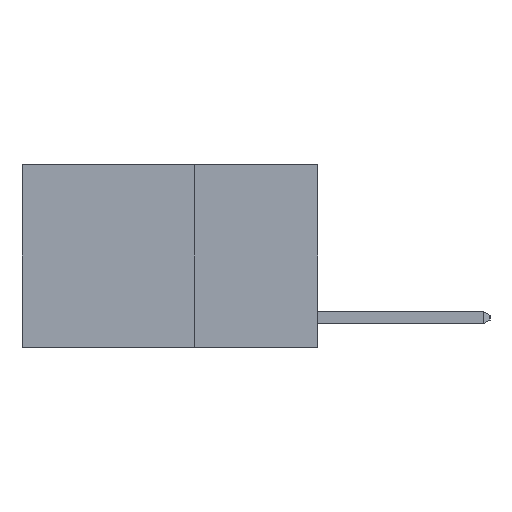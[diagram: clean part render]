
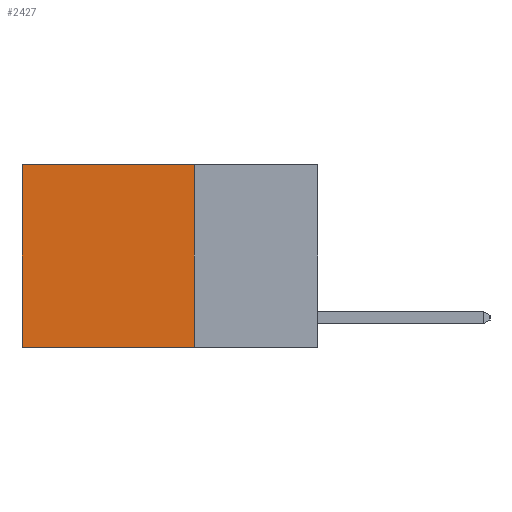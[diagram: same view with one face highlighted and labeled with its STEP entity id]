
A CAD part, left-side view. The second image highlights one B-rep face of the part: STEP entity #2427.
In plain terms, the highlighted planar face has unit normal (-1, 0, 0).
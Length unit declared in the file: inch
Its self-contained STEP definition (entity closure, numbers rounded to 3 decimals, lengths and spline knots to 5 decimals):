
#36 = VERTEX_POINT ( 'NONE', #8990 ) ;
#285 = CARTESIAN_POINT ( 'NONE',  ( 0.2625, 0.6, 0. ) ) ;
#455 = CARTESIAN_POINT ( 'NONE',  ( 0.2625, 0.25, 0. ) ) ;
#501 = EDGE_CURVE ( 'NONE', #3839, #36, #5821, .T. ) ;
#644 = VERTEX_POINT ( 'NONE', #3275 ) ;
#1100 = CARTESIAN_POINT ( 'NONE',  ( 0.2625, 0.25, 0. ) ) ;
#1375 = EDGE_CURVE ( 'NONE', #2081, #644, #3264, .T. ) ;
#1505 = VECTOR ( 'NONE', #6286, 39.37008 ) ;
#1747 = CARTESIAN_POINT ( 'NONE',  ( 0.2625, 0.25, 0. ) ) ;
#1783 = CARTESIAN_POINT ( 'NONE',  ( 0.2625, 0.6, 0. ) ) ;
#1934 = DIRECTION ( 'NONE',  ( 0., 1., 0. ) ) ;
#2081 = VERTEX_POINT ( 'NONE', #5752 ) ;
#2155 = LINE ( 'NONE', #1100, #7421 ) ;
#2427 = ADVANCED_FACE ( 'NONE', ( #4930 ), #5944, .F. ) ;
#2529 = ORIENTED_EDGE ( 'NONE', *, *, #2788, .F. ) ;
#2567 = ORIENTED_EDGE ( 'NONE', *, *, #501, .T. ) ;
#2575 = DIRECTION ( 'NONE',  ( 0., 0., -1. ) ) ;
#2788 = EDGE_CURVE ( 'NONE', #644, #36, #6197, .T. ) ;
#2846 = DIRECTION ( 'NONE',  ( 0., 0., -1. ) ) ;
#3264 = LINE ( 'NONE', #455, #1505 ) ;
#3275 = CARTESIAN_POINT ( 'NONE',  ( 0.2625, 0.25, -0.37 ) ) ;
#3599 = ORIENTED_EDGE ( 'NONE', *, *, #1375, .F. ) ;
#3839 = VERTEX_POINT ( 'NONE', #285 ) ;
#4930 = FACE_OUTER_BOUND ( 'NONE', #6091, .T. ) ;
#5655 = CARTESIAN_POINT ( 'NONE',  ( 0.2625, 0.25, -0.37 ) ) ;
#5752 = CARTESIAN_POINT ( 'NONE',  ( 0.2625, 0.25, 0. ) ) ;
#5821 = LINE ( 'NONE', #1783, #8432 ) ;
#5944 = PLANE ( 'NONE',  #6532 ) ;
#6091 = EDGE_LOOP ( 'NONE', ( #2567, #2529, #3599, #7225 ) ) ;
#6130 = EDGE_CURVE ( 'NONE', #2081, #3839, #2155, .T. ) ;
#6197 = LINE ( 'NONE', #5655, #7818 ) ;
#6286 = DIRECTION ( 'NONE',  ( 0., 0., -1. ) ) ;
#6532 = AXIS2_PLACEMENT_3D ( 'NONE', #1747, #6651, #2575 ) ;
#6651 = DIRECTION ( 'NONE',  ( 1., 0., 0. ) ) ;
#7225 = ORIENTED_EDGE ( 'NONE', *, *, #6130, .T. ) ;
#7421 = VECTOR ( 'NONE', #1934, 39.37008 ) ;
#7739 = DIRECTION ( 'NONE',  ( 0., 1., 0. ) ) ;
#7818 = VECTOR ( 'NONE', #7739, 39.37008 ) ;
#8432 = VECTOR ( 'NONE', #2846, 39.37008 ) ;
#8990 = CARTESIAN_POINT ( 'NONE',  ( 0.2625, 0.6, -0.37 ) ) ;
